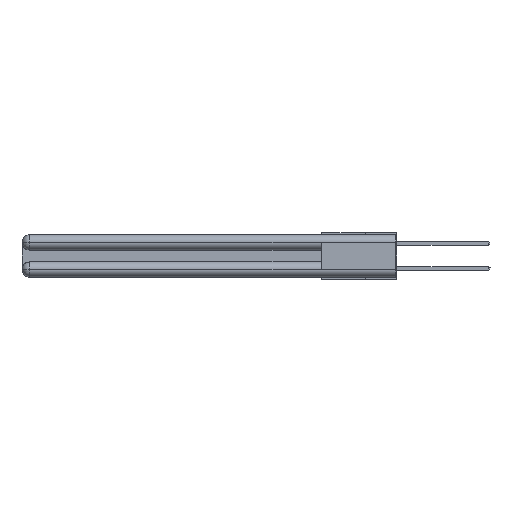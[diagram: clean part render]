
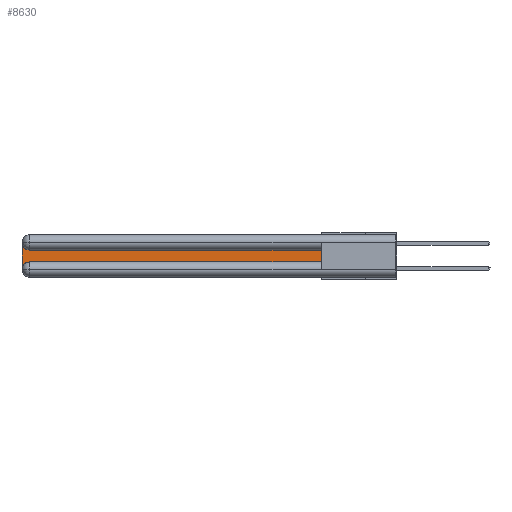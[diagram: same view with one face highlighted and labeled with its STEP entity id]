
A CAD part, left-side view. The second image highlights one B-rep face of the part: STEP entity #8630.
In plain terms, the highlighted planar face has unit normal (-1, 0, 0).
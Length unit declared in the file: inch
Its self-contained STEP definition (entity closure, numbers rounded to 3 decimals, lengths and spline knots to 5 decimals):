
#366 = DIRECTION ( 'NONE',  ( 1., 0., 0. ) ) ;
#864 = LINE ( 'NONE', #18650, #4103 ) ;
#1190 = CARTESIAN_POINT ( 'NONE',  ( 0.075, 2.94, -0.1225 ) ) ;
#1290 = DIRECTION ( 'NONE',  ( 0., 0., -1. ) ) ;
#1824 = AXIS2_PLACEMENT_3D ( 'NONE', #19466, #26475, #5602 ) ;
#2233 = CARTESIAN_POINT ( 'NONE',  ( 0.075, 3., -0.2775 ) ) ;
#2604 = CARTESIAN_POINT ( 'NONE',  ( 0.075, 2.94, -0.0625 ) ) ;
#3461 = EDGE_CURVE ( 'NONE', #14195, #13573, #20653, .T. ) ;
#3522 = DIRECTION ( 'NONE',  ( 0., 1., 0. ) ) ;
#4103 = VECTOR ( 'NONE', #7233, 39.37008 ) ;
#4226 = VECTOR ( 'NONE', #5928, 39.37008 ) ;
#4878 = VERTEX_POINT ( 'NONE', #2233 ) ;
#5602 = DIRECTION ( 'NONE',  ( 0., 0., -1. ) ) ;
#5928 = DIRECTION ( 'NONE',  ( 0., 0., 1. ) ) ;
#5991 = CARTESIAN_POINT ( 'NONE',  ( 0.075, 0.6, -0.1225 ) ) ;
#7233 = DIRECTION ( 'NONE',  ( 0., -1., 0. ) ) ;
#7533 = ORIENTED_EDGE ( 'NONE', *, *, #27803, .T. ) ;
#8630 = ADVANCED_FACE ( 'NONE', ( #16340 ), #10738, .F. ) ;
#8647 = CARTESIAN_POINT ( 'NONE',  ( 0.075, 0.6, -0.2175 ) ) ;
#9591 = LINE ( 'NONE', #8647, #4226 ) ;
#10738 = PLANE ( 'NONE',  #18078 ) ;
#10792 = DIRECTION ( 'NONE',  ( 0., 0., -1. ) ) ;
#10836 = ORIENTED_EDGE ( 'NONE', *, *, #20118, .T. ) ;
#11778 = ORIENTED_EDGE ( 'NONE', *, *, #18954, .T. ) ;
#12764 = DIRECTION ( 'NONE',  ( 1., 0., 0. ) ) ;
#13062 = CARTESIAN_POINT ( 'NONE',  ( 0.075, 3., -0.1225 ) ) ;
#13573 = VERTEX_POINT ( 'NONE', #25876 ) ;
#13575 = VECTOR ( 'NONE', #3522, 39.37008 ) ;
#13668 = LINE ( 'NONE', #24060, #24555 ) ;
#14195 = VERTEX_POINT ( 'NONE', #1190 ) ;
#15832 = VERTEX_POINT ( 'NONE', #26325 ) ;
#16340 = FACE_OUTER_BOUND ( 'NONE', #27504, .T. ) ;
#17683 = CIRCLE ( 'NONE', #1824, 0.06 ) ;
#18078 = AXIS2_PLACEMENT_3D ( 'NONE', #13062, #12764, #1290 ) ;
#18650 = CARTESIAN_POINT ( 'NONE',  ( 0.075, 0.6, -0.2175 ) ) ;
#18954 = EDGE_CURVE ( 'NONE', #13573, #4878, #13668, .T. ) ;
#19338 = LINE ( 'NONE', #5991, #13575 ) ;
#19466 = CARTESIAN_POINT ( 'NONE',  ( 0.075, 2.94, -0.2775 ) ) ;
#19984 = AXIS2_PLACEMENT_3D ( 'NONE', #2604, #366, #28338 ) ;
#20118 = EDGE_CURVE ( 'NONE', #20869, #15832, #9591, .T. ) ;
#20346 = CARTESIAN_POINT ( 'NONE',  ( 0.075, 2.94, -0.2175 ) ) ;
#20364 = ORIENTED_EDGE ( 'NONE', *, *, #26394, .T. ) ;
#20653 = CIRCLE ( 'NONE', #19984, 0.06 ) ;
#20690 = ORIENTED_EDGE ( 'NONE', *, *, #20801, .T. ) ;
#20801 = EDGE_CURVE ( 'NONE', #15832, #14195, #19338, .T. ) ;
#20869 = VERTEX_POINT ( 'NONE', #24524 ) ;
#22029 = ORIENTED_EDGE ( 'NONE', *, *, #3461, .T. ) ;
#24060 = CARTESIAN_POINT ( 'NONE',  ( 0.075, 3., -0.2175 ) ) ;
#24524 = CARTESIAN_POINT ( 'NONE',  ( 0.075, 0.6, -0.2175 ) ) ;
#24555 = VECTOR ( 'NONE', #10792, 39.37008 ) ;
#25876 = CARTESIAN_POINT ( 'NONE',  ( 0.075, 3., -0.0625 ) ) ;
#26250 = VERTEX_POINT ( 'NONE', #20346 ) ;
#26325 = CARTESIAN_POINT ( 'NONE',  ( 0.075, 0.6, -0.1225 ) ) ;
#26394 = EDGE_CURVE ( 'NONE', #26250, #20869, #864, .T. ) ;
#26475 = DIRECTION ( 'NONE',  ( 1., 0., 0. ) ) ;
#27504 = EDGE_LOOP ( 'NONE', ( #20690, #22029, #11778, #7533, #20364, #10836 ) ) ;
#27803 = EDGE_CURVE ( 'NONE', #4878, #26250, #17683, .T. ) ;
#28338 = DIRECTION ( 'NONE',  ( 0., 0., -1. ) ) ;
